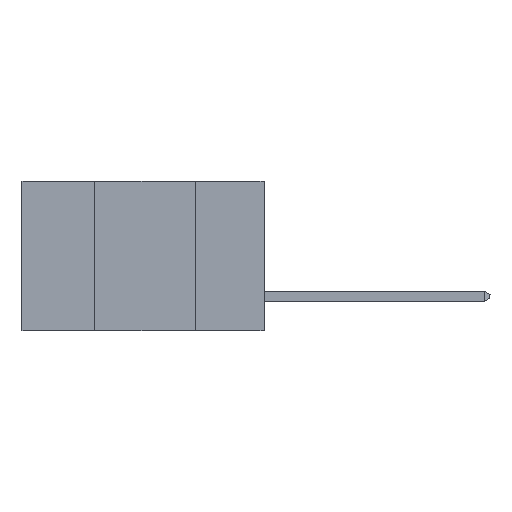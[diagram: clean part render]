
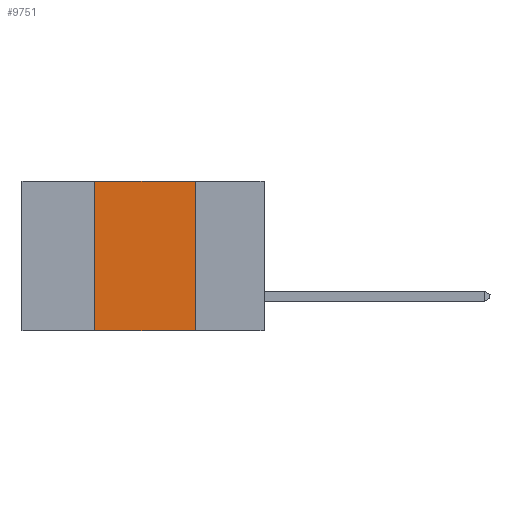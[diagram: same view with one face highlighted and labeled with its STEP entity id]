
A CAD part, left-side view. The second image highlights one B-rep face of the part: STEP entity #9751.
In plain terms, the highlighted planar face has unit normal (-1, 0, 0).
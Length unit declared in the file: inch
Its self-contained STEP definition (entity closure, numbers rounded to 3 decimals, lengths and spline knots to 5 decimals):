
#926 = AXIS2_PLACEMENT_3D ( 'NONE', #20676, #14691, #10666 ) ;
#979 = LINE ( 'NONE', #1055, #16279 ) ;
#1055 = CARTESIAN_POINT ( 'NONE',  ( 0., 0.17, 0. ) ) ;
#1137 = ORIENTED_EDGE ( 'NONE', *, *, #1738, .F. ) ;
#1738 = EDGE_CURVE ( 'NONE', #23105, #10120, #979, .T. ) ;
#3748 = DIRECTION ( 'NONE',  ( 0., -1., 0. ) ) ;
#3908 = EDGE_CURVE ( 'NONE', #10349, #10120, #22727, .T. ) ;
#4222 = VERTEX_POINT ( 'NONE', #4383 ) ;
#4383 = CARTESIAN_POINT ( 'NONE',  ( 0., 0.42, 0. ) ) ;
#4916 = CARTESIAN_POINT ( 'NONE',  ( 0., 0.42, -0.37 ) ) ;
#5016 = CARTESIAN_POINT ( 'NONE',  ( 0., 0.17, -0.37 ) ) ;
#5691 = ORIENTED_EDGE ( 'NONE', *, *, #3908, .T. ) ;
#6746 = VECTOR ( 'NONE', #20829, 39.37008 ) ;
#8312 = VECTOR ( 'NONE', #3748, 39.37008 ) ;
#9199 = ORIENTED_EDGE ( 'NONE', *, *, #23830, .F. ) ;
#9751 = ADVANCED_FACE ( 'NONE', ( #11890 ), #18678, .F. ) ;
#10120 = VERTEX_POINT ( 'NONE', #5016 ) ;
#10216 = EDGE_LOOP ( 'NONE', ( #1137, #15617, #9199, #5691 ) ) ;
#10349 = VERTEX_POINT ( 'NONE', #4916 ) ;
#10666 = DIRECTION ( 'NONE',  ( 0., 0., -1. ) ) ;
#10886 = LINE ( 'NONE', #25838, #8312 ) ;
#10918 = DIRECTION ( 'NONE',  ( 0., 0., -1. ) ) ;
#11890 = FACE_OUTER_BOUND ( 'NONE', #10216, .T. ) ;
#13980 = CARTESIAN_POINT ( 'NONE',  ( 0., 0.42, 0. ) ) ;
#14229 = VECTOR ( 'NONE', #23738, 39.37008 ) ;
#14468 = EDGE_CURVE ( 'NONE', #4222, #23105, #10886, .T. ) ;
#14691 = DIRECTION ( 'NONE',  ( 1., 0., 0. ) ) ;
#15617 = ORIENTED_EDGE ( 'NONE', *, *, #14468, .F. ) ;
#16279 = VECTOR ( 'NONE', #10918, 39.37008 ) ;
#17014 = CARTESIAN_POINT ( 'NONE',  ( 0., 0.6, -0.37 ) ) ;
#18678 = PLANE ( 'NONE',  #926 ) ;
#20134 = LINE ( 'NONE', #13980, #14229 ) ;
#20676 = CARTESIAN_POINT ( 'NONE',  ( 0., 0.6, 0. ) ) ;
#20829 = DIRECTION ( 'NONE',  ( 0., -1., 0. ) ) ;
#22727 = LINE ( 'NONE', #17014, #6746 ) ;
#23105 = VERTEX_POINT ( 'NONE', #25614 ) ;
#23738 = DIRECTION ( 'NONE',  ( 0., 0., 1. ) ) ;
#23830 = EDGE_CURVE ( 'NONE', #10349, #4222, #20134, .T. ) ;
#25614 = CARTESIAN_POINT ( 'NONE',  ( 0., 0.17, 0. ) ) ;
#25838 = CARTESIAN_POINT ( 'NONE',  ( 0., 0.6, 0. ) ) ;
